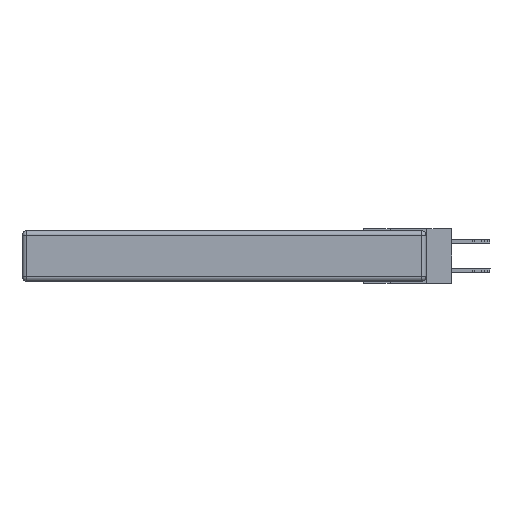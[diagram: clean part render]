
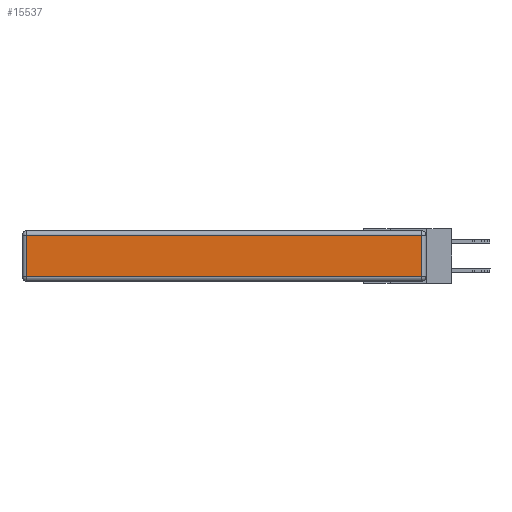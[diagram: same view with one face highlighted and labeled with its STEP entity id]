
A CAD part, left-side view. The second image highlights one B-rep face of the part: STEP entity #15537.
In plain terms, the highlighted planar face has unit normal (-1, 0, 0).
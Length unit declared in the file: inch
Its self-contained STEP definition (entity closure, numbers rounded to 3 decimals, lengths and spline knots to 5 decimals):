
#478 = DIRECTION ( 'NONE',  ( -1., 0., 0. ) ) ;
#2163 = DIRECTION ( 'NONE',  ( 0., -1., 0. ) ) ;
#3200 = DIRECTION ( 'NONE',  ( 0., 0., 1. ) ) ;
#4433 = EDGE_CURVE ( 'NONE', #16553, #4718, #9760, .T. ) ;
#4491 = AXIS2_PLACEMENT_3D ( 'NONE', #8028, #478, #3200 ) ;
#4614 = CARTESIAN_POINT ( 'NONE',  ( 0., 2.72, -0.313 ) ) ;
#4718 = VERTEX_POINT ( 'NONE', #19656 ) ;
#5257 = ORIENTED_EDGE ( 'NONE', *, *, #4433, .T. ) ;
#5868 = ORIENTED_EDGE ( 'NONE', *, *, #20076, .T. ) ;
#6340 = DIRECTION ( 'NONE',  ( 0., 0., 1. ) ) ;
#7543 = VECTOR ( 'NONE', #6340, 39.37008 ) ;
#8028 = CARTESIAN_POINT ( 'NONE',  ( 0., 0., -0.343 ) ) ;
#8319 = VECTOR ( 'NONE', #10420, 39.37008 ) ;
#8468 = ORIENTED_EDGE ( 'NONE', *, *, #18529, .T. ) ;
#8835 = CARTESIAN_POINT ( 'NONE',  ( 0., 2.72, -0.343 ) ) ;
#8863 = VERTEX_POINT ( 'NONE', #19680 ) ;
#8938 = DIRECTION ( 'NONE',  ( 0., 0., -1. ) ) ;
#9760 = LINE ( 'NONE', #20912, #19406 ) ;
#10420 = DIRECTION ( 'NONE',  ( 0., 1., 0. ) ) ;
#13123 = VECTOR ( 'NONE', #8938, 39.37008 ) ;
#13797 = EDGE_LOOP ( 'NONE', ( #5257, #5868, #14146, #8468 ) ) ;
#14146 = ORIENTED_EDGE ( 'NONE', *, *, #18348, .T. ) ;
#14577 = LINE ( 'NONE', #27381, #7543 ) ;
#14868 = PLANE ( 'NONE',  #4491 ) ;
#15537 = ADVANCED_FACE ( 'NONE', ( #26777 ), #14868, .T. ) ;
#16553 = VERTEX_POINT ( 'NONE', #4614 ) ;
#16991 = CARTESIAN_POINT ( 'NONE',  ( 0., 0.03, -0.03 ) ) ;
#18348 = EDGE_CURVE ( 'NONE', #26908, #8863, #20216, .T. ) ;
#18529 = EDGE_CURVE ( 'NONE', #8863, #16553, #26563, .T. ) ;
#19406 = VECTOR ( 'NONE', #2163, 39.37008 ) ;
#19656 = CARTESIAN_POINT ( 'NONE',  ( 0., 0.03, -0.313 ) ) ;
#19680 = CARTESIAN_POINT ( 'NONE',  ( 0., 2.72, -0.03 ) ) ;
#20076 = EDGE_CURVE ( 'NONE', #4718, #26908, #14577, .T. ) ;
#20216 = LINE ( 'NONE', #27272, #8319 ) ;
#20912 = CARTESIAN_POINT ( 'NONE',  ( 0., 0., -0.313 ) ) ;
#26563 = LINE ( 'NONE', #8835, #13123 ) ;
#26777 = FACE_OUTER_BOUND ( 'NONE', #13797, .T. ) ;
#26908 = VERTEX_POINT ( 'NONE', #16991 ) ;
#27272 = CARTESIAN_POINT ( 'NONE',  ( 0., 2.75, -0.03 ) ) ;
#27381 = CARTESIAN_POINT ( 'NONE',  ( 0., 0.03, -0.343 ) ) ;
